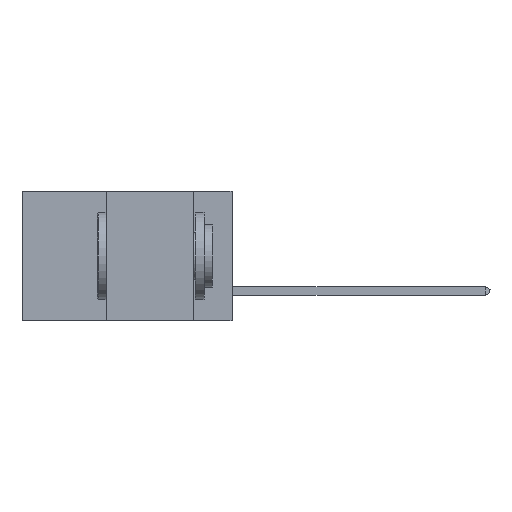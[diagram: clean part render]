
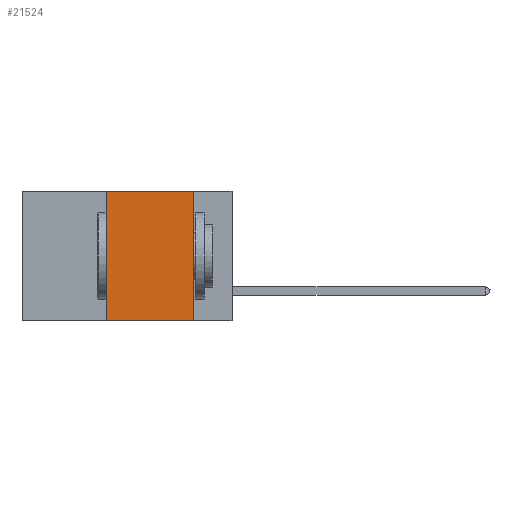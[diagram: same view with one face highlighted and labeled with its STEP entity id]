
A CAD part, left-side view. The second image highlights one B-rep face of the part: STEP entity #21524.
In plain terms, the highlighted planar face has unit normal (-1, 0, 0).
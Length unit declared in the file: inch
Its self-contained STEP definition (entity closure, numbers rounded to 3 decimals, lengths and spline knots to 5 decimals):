
#940 = VERTEX_POINT ( 'NONE', #23471 ) ;
#1194 = CARTESIAN_POINT ( 'NONE',  ( 0., 0.36, 0. ) ) ;
#1893 = CARTESIAN_POINT ( 'NONE',  ( 0., 0.11, -0.37 ) ) ;
#2328 = LINE ( 'NONE', #19742, #15026 ) ;
#2534 = FACE_OUTER_BOUND ( 'NONE', #13926, .T. ) ;
#3146 = DIRECTION ( 'NONE',  ( 0., 0., -1. ) ) ;
#3340 = CARTESIAN_POINT ( 'NONE',  ( 0., 0.11, 0. ) ) ;
#3354 = VERTEX_POINT ( 'NONE', #1893 ) ;
#5408 = ORIENTED_EDGE ( 'NONE', *, *, #24797, .F. ) ;
#5603 = VECTOR ( 'NONE', #23821, 39.37008 ) ;
#6619 = VECTOR ( 'NONE', #22926, 39.37008 ) ;
#6709 = CARTESIAN_POINT ( 'NONE',  ( 0., 0.36, -0.37 ) ) ;
#7417 = ORIENTED_EDGE ( 'NONE', *, *, #13999, .F. ) ;
#7856 = DIRECTION ( 'NONE',  ( 0., -1., 0. ) ) ;
#8626 = DIRECTION ( 'NONE',  ( 1., 0., 0. ) ) ;
#8925 = LINE ( 'NONE', #3340, #22918 ) ;
#9000 = LINE ( 'NONE', #15997, #5603 ) ;
#10255 = EDGE_CURVE ( 'NONE', #18762, #3354, #2328, .T. ) ;
#10764 = ORIENTED_EDGE ( 'NONE', *, *, #12505, .F. ) ;
#11886 = LINE ( 'NONE', #1194, #6619 ) ;
#12505 = EDGE_CURVE ( 'NONE', #940, #19063, #9000, .T. ) ;
#13926 = EDGE_LOOP ( 'NONE', ( #7417, #10764, #5408, #17364 ) ) ;
#13999 = EDGE_CURVE ( 'NONE', #19063, #3354, #8925, .T. ) ;
#14467 = CARTESIAN_POINT ( 'NONE',  ( 0., 0.11, 0. ) ) ;
#15026 = VECTOR ( 'NONE', #7856, 39.37008 ) ;
#15997 = CARTESIAN_POINT ( 'NONE',  ( 0., 0.6, 0. ) ) ;
#16511 = DIRECTION ( 'NONE',  ( 0., 0., -1. ) ) ;
#17364 = ORIENTED_EDGE ( 'NONE', *, *, #10255, .T. ) ;
#18762 = VERTEX_POINT ( 'NONE', #6709 ) ;
#19063 = VERTEX_POINT ( 'NONE', #14467 ) ;
#19742 = CARTESIAN_POINT ( 'NONE',  ( 0., 0.6, -0.37 ) ) ;
#20579 = CARTESIAN_POINT ( 'NONE',  ( 0., 0.6, 0. ) ) ;
#20924 = AXIS2_PLACEMENT_3D ( 'NONE', #20579, #8626, #16511 ) ;
#21524 = ADVANCED_FACE ( 'NONE', ( #2534 ), #24369, .F. ) ;
#22918 = VECTOR ( 'NONE', #3146, 39.37008 ) ;
#22926 = DIRECTION ( 'NONE',  ( 0., 0., 1. ) ) ;
#23471 = CARTESIAN_POINT ( 'NONE',  ( 0., 0.36, 0. ) ) ;
#23821 = DIRECTION ( 'NONE',  ( 0., -1., 0. ) ) ;
#24369 = PLANE ( 'NONE',  #20924 ) ;
#24797 = EDGE_CURVE ( 'NONE', #18762, #940, #11886, .T. ) ;
